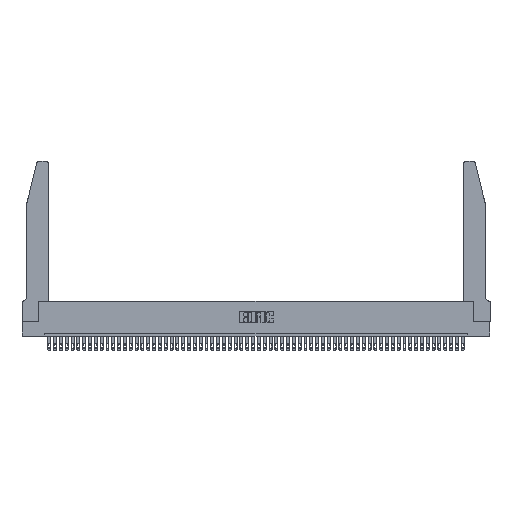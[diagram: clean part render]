
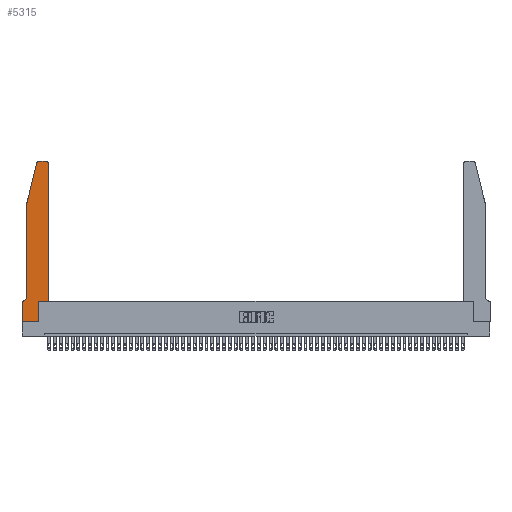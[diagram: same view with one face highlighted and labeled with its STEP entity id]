
A CAD part, top view. The second image highlights one B-rep face of the part: STEP entity #5315.
In plain terms, the highlighted planar face has unit normal (0, 0, 1).
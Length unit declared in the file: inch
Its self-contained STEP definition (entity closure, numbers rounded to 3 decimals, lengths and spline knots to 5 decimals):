
#181 = CARTESIAN_POINT ( 'NONE',  ( 0.2865, 0.35, 0.37 ) ) ;
#651 = ORIENTED_EDGE ( 'NONE', *, *, #18202, .T. ) ;
#874 = DIRECTION ( 'NONE',  ( -1., 0., 0. ) ) ;
#1284 = VERTEX_POINT ( 'NONE', #42062 ) ;
#1356 = CARTESIAN_POINT ( 'NONE',  ( 0.0755, 2., 0.37 ) ) ;
#2296 = CARTESIAN_POINT ( 'NONE',  ( 0.0755, 2., 0.37 ) ) ;
#2340 = EDGE_CURVE ( 'NONE', #1284, #5762, #44422, .T. ) ;
#2957 = VERTEX_POINT ( 'NONE', #35855 ) ;
#3430 = DIRECTION ( 'NONE',  ( 0., 0., 1. ) ) ;
#3952 = ORIENTED_EDGE ( 'NONE', *, *, #46983, .T. ) ;
#4178 = EDGE_CURVE ( 'NONE', #43251, #13596, #50255, .T. ) ;
#4274 = VECTOR ( 'NONE', #26547, 39.37008 ) ;
#5315 = ADVANCED_FACE ( 'NONE', ( #13073 ), #7269, .T. ) ;
#5663 = CARTESIAN_POINT ( 'NONE',  ( 0.4505, 0.35, 0.37 ) ) ;
#5762 = VERTEX_POINT ( 'NONE', #16552 ) ;
#6675 = CARTESIAN_POINT ( 'NONE',  ( 0.284, 2.72, 0.37 ) ) ;
#7269 = PLANE ( 'NONE',  #26146 ) ;
#7835 = CIRCLE ( 'NONE', #35542, 0.07 ) ;
#8295 = VERTEX_POINT ( 'NONE', #54669 ) ;
#9287 = VECTOR ( 'NONE', #48612, 39.37008 ) ;
#9470 = DIRECTION ( 'NONE',  ( 0., 0., -1. ) ) ;
#9634 = LINE ( 'NONE', #30126, #53425 ) ;
#9954 = CARTESIAN_POINT ( 'NONE',  ( 0., 0., 0.37 ) ) ;
#10664 = DIRECTION ( 'NONE',  ( 1., 0., 0. ) ) ;
#11719 = VERTEX_POINT ( 'NONE', #15506 ) ;
#11928 = DIRECTION ( 'NONE',  ( 1., 0., 0. ) ) ;
#12416 = ORIENTED_EDGE ( 'NONE', *, *, #41523, .T. ) ;
#12527 = EDGE_CURVE ( 'NONE', #13596, #1284, #25777, .T. ) ;
#12643 = CARTESIAN_POINT ( 'NONE',  ( 0., 0.35, 0.37 ) ) ;
#13073 = FACE_OUTER_BOUND ( 'NONE', #38850, .T. ) ;
#13596 = VERTEX_POINT ( 'NONE', #40497 ) ;
#13712 = DIRECTION ( 'NONE',  ( -1., 0., 0. ) ) ;
#13924 = EDGE_CURVE ( 'NONE', #41258, #54685, #45524, .T. ) ;
#14558 = DIRECTION ( 'NONE',  ( 0., 1., 0. ) ) ;
#14949 = DIRECTION ( 'NONE',  ( 1., 0., 0. ) ) ;
#15121 = DIRECTION ( 'NONE',  ( -1., 0., 0. ) ) ;
#15506 = CARTESIAN_POINT ( 'NONE',  ( 0.25487, 2.72718, 0.37 ) ) ;
#15874 = CIRCLE ( 'NONE', #21222, 0.03 ) ;
#16552 = CARTESIAN_POINT ( 'NONE',  ( 0.284, 2.75, 0.37 ) ) ;
#18202 = EDGE_CURVE ( 'NONE', #28035, #41258, #20613, .T. ) ;
#18306 = DIRECTION ( 'NONE',  ( 0., 1., 0. ) ) ;
#20247 = CARTESIAN_POINT ( 'NONE',  ( 0.4205, 2.72, 0.37 ) ) ;
#20613 = LINE ( 'NONE', #39367, #9287 ) ;
#21063 = VERTEX_POINT ( 'NONE', #12643 ) ;
#21222 = AXIS2_PLACEMENT_3D ( 'NONE', #6675, #23242, #14949 ) ;
#22565 = EDGE_CURVE ( 'NONE', #8295, #50656, #7835, .T. ) ;
#22964 = DIRECTION ( 'NONE',  ( 0., -1., 0. ) ) ;
#23242 = DIRECTION ( 'NONE',  ( 0., 0., 1. ) ) ;
#23414 = ORIENTED_EDGE ( 'NONE', *, *, #12527, .T. ) ;
#24279 = EDGE_CURVE ( 'NONE', #11719, #2957, #39229, .T. ) ;
#24382 = ORIENTED_EDGE ( 'NONE', *, *, #28419, .T. ) ;
#24562 = ORIENTED_EDGE ( 'NONE', *, *, #29777, .T. ) ;
#25777 = CIRCLE ( 'NONE', #48677, 0.03 ) ;
#26022 = LINE ( 'NONE', #2296, #39275 ) ;
#26146 = AXIS2_PLACEMENT_3D ( 'NONE', #36006, #41058, #10664 ) ;
#26182 = DIRECTION ( 'NONE',  ( 1., 0., 0. ) ) ;
#26547 = DIRECTION ( 'NONE',  ( -0.239, -0.971, 0. ) ) ;
#28035 = VERTEX_POINT ( 'NONE', #9954 ) ;
#28419 = EDGE_CURVE ( 'NONE', #2957, #8295, #26022, .T. ) ;
#28725 = CARTESIAN_POINT ( 'NONE',  ( 0.4505, 0.35, 0.37 ) ) ;
#29678 = VECTOR ( 'NONE', #18306, 39.37008 ) ;
#29777 = EDGE_CURVE ( 'NONE', #21063, #28035, #54474, .T. ) ;
#30126 = CARTESIAN_POINT ( 'NONE',  ( 0.4505, 0.35, 0.37 ) ) ;
#32169 = CARTESIAN_POINT ( 'NONE',  ( 0., 0., 0.37 ) ) ;
#33006 = VECTOR ( 'NONE', #15121, 39.37008 ) ;
#34321 = ORIENTED_EDGE ( 'NONE', *, *, #24279, .T. ) ;
#35542 = AXIS2_PLACEMENT_3D ( 'NONE', #39049, #9470, #13712 ) ;
#35855 = CARTESIAN_POINT ( 'NONE',  ( 0.0755, 2., 0.37 ) ) ;
#35992 = CARTESIAN_POINT ( 'NONE',  ( 0.0755, 0.35, 0.37 ) ) ;
#36006 = CARTESIAN_POINT ( 'NONE',  ( 0., 0.35, 0.37 ) ) ;
#36617 = DIRECTION ( 'NONE',  ( 0., -1., 0. ) ) ;
#38429 = ORIENTED_EDGE ( 'NONE', *, *, #22565, .T. ) ;
#38850 = EDGE_LOOP ( 'NONE', ( #52345, #12416, #34321, #24382, #38429, #43629, #24562, #651, #47828, #3952, #54177, #23414 ) ) ;
#38905 = VECTOR ( 'NONE', #14558, 39.37008 ) ;
#39049 = CARTESIAN_POINT ( 'NONE',  ( 0.0055, 0.42, 0.37 ) ) ;
#39229 = LINE ( 'NONE', #1356, #4274 ) ;
#39275 = VECTOR ( 'NONE', #22964, 39.37008 ) ;
#39367 = CARTESIAN_POINT ( 'NONE',  ( 0., 0., 0.37 ) ) ;
#39459 = CARTESIAN_POINT ( 'NONE',  ( 0.0055, 0.35, 0.37 ) ) ;
#40497 = CARTESIAN_POINT ( 'NONE',  ( 0.4505, 2.72, 0.37 ) ) ;
#41058 = DIRECTION ( 'NONE',  ( 0., 0., 1. ) ) ;
#41258 = VERTEX_POINT ( 'NONE', #51196 ) ;
#41523 = EDGE_CURVE ( 'NONE', #5762, #11719, #15874, .T. ) ;
#41872 = VECTOR ( 'NONE', #874, 39.37008 ) ;
#42062 = CARTESIAN_POINT ( 'NONE',  ( 0.4205, 2.75, 0.37 ) ) ;
#42613 = CARTESIAN_POINT ( 'NONE',  ( 0.2865, 0.35, 0.37 ) ) ;
#43251 = VERTEX_POINT ( 'NONE', #28725 ) ;
#43629 = ORIENTED_EDGE ( 'NONE', *, *, #45807, .T. ) ;
#44367 = VECTOR ( 'NONE', #36617, 39.37008 ) ;
#44422 = LINE ( 'NONE', #50714, #41872 ) ;
#45524 = LINE ( 'NONE', #42613, #29678 ) ;
#45807 = EDGE_CURVE ( 'NONE', #50656, #21063, #49520, .T. ) ;
#46983 = EDGE_CURVE ( 'NONE', #54685, #43251, #9634, .T. ) ;
#47828 = ORIENTED_EDGE ( 'NONE', *, *, #13924, .T. ) ;
#48612 = DIRECTION ( 'NONE',  ( 1., 0., 0. ) ) ;
#48677 = AXIS2_PLACEMENT_3D ( 'NONE', #20247, #3430, #11928 ) ;
#49520 = LINE ( 'NONE', #35992, #33006 ) ;
#50255 = LINE ( 'NONE', #5663, #38905 ) ;
#50656 = VERTEX_POINT ( 'NONE', #39459 ) ;
#50714 = CARTESIAN_POINT ( 'NONE',  ( 0.2605, 2.75, 0.37 ) ) ;
#51196 = CARTESIAN_POINT ( 'NONE',  ( 0.2865, 0., 0.37 ) ) ;
#52345 = ORIENTED_EDGE ( 'NONE', *, *, #2340, .T. ) ;
#53425 = VECTOR ( 'NONE', #26182, 39.37008 ) ;
#54177 = ORIENTED_EDGE ( 'NONE', *, *, #4178, .T. ) ;
#54474 = LINE ( 'NONE', #32169, #44367 ) ;
#54669 = CARTESIAN_POINT ( 'NONE',  ( 0.0755, 0.42, 0.37 ) ) ;
#54685 = VERTEX_POINT ( 'NONE', #181 ) ;
